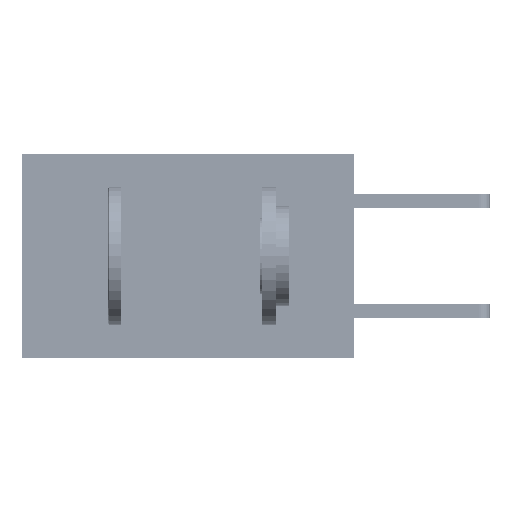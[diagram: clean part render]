
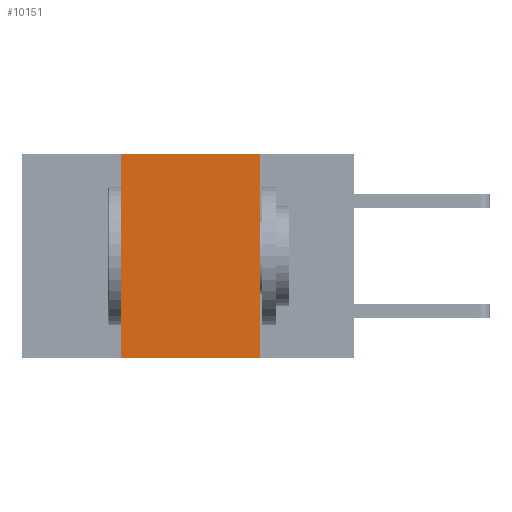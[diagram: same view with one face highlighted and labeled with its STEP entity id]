
A CAD part, left-side view. The second image highlights one B-rep face of the part: STEP entity #10151.
In plain terms, the highlighted planar face has unit normal (-1, 0, 0).
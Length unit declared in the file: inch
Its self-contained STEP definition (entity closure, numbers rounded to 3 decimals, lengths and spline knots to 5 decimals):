
#2378 = LINE ( 'NONE', #46864, #11635 ) ;
#2571 = VECTOR ( 'NONE', #17603, 39.37008 ) ;
#6655 = DIRECTION ( 'NONE',  ( 0., 0., 1. ) ) ;
#6708 = VECTOR ( 'NONE', #42373, 39.37008 ) ;
#7943 = LINE ( 'NONE', #14848, #24016 ) ;
#8687 = AXIS2_PLACEMENT_3D ( 'NONE', #32203, #43185, #32829 ) ;
#9310 = EDGE_CURVE ( 'NONE', #33390, #25339, #2378, .T. ) ;
#10151 = ADVANCED_FACE ( 'NONE', ( #14935 ), #24885, .F. ) ;
#10467 = ORIENTED_EDGE ( 'NONE', *, *, #22022, .F. ) ;
#10662 = CARTESIAN_POINT ( 'NONE',  ( 0., 0.42, 0. ) ) ;
#11635 = VECTOR ( 'NONE', #6655, 39.37008 ) ;
#14848 = CARTESIAN_POINT ( 'NONE',  ( 0., 0.17, 0. ) ) ;
#14935 = FACE_OUTER_BOUND ( 'NONE', #37610, .T. ) ;
#15115 = ORIENTED_EDGE ( 'NONE', *, *, #21054, .F. ) ;
#17018 = CARTESIAN_POINT ( 'NONE',  ( 0., 0.6, 0. ) ) ;
#17603 = DIRECTION ( 'NONE',  ( 0., -1., 0. ) ) ;
#21054 = EDGE_CURVE ( 'NONE', #28473, #40929, #7943, .T. ) ;
#21909 = DIRECTION ( 'NONE',  ( 0., 0., -1. ) ) ;
#22022 = EDGE_CURVE ( 'NONE', #25339, #28473, #27363, .T. ) ;
#24016 = VECTOR ( 'NONE', #21909, 39.37008 ) ;
#24484 = CARTESIAN_POINT ( 'NONE',  ( 0., 0.6, -0.37 ) ) ;
#24885 = PLANE ( 'NONE',  #8687 ) ;
#25339 = VERTEX_POINT ( 'NONE', #10662 ) ;
#27363 = LINE ( 'NONE', #17018, #6708 ) ;
#28473 = VERTEX_POINT ( 'NONE', #30094 ) ;
#29717 = ORIENTED_EDGE ( 'NONE', *, *, #37315, .T. ) ;
#30094 = CARTESIAN_POINT ( 'NONE',  ( 0., 0.17, 0. ) ) ;
#31801 = LINE ( 'NONE', #24484, #2571 ) ;
#32203 = CARTESIAN_POINT ( 'NONE',  ( 0., 0.6, 0. ) ) ;
#32829 = DIRECTION ( 'NONE',  ( 0., 0., -1. ) ) ;
#33390 = VERTEX_POINT ( 'NONE', #35704 ) ;
#34138 = ORIENTED_EDGE ( 'NONE', *, *, #9310, .F. ) ;
#35704 = CARTESIAN_POINT ( 'NONE',  ( 0., 0.42, -0.37 ) ) ;
#37315 = EDGE_CURVE ( 'NONE', #33390, #40929, #31801, .T. ) ;
#37610 = EDGE_LOOP ( 'NONE', ( #15115, #10467, #34138, #29717 ) ) ;
#40929 = VERTEX_POINT ( 'NONE', #45822 ) ;
#42373 = DIRECTION ( 'NONE',  ( 0., -1., 0. ) ) ;
#43185 = DIRECTION ( 'NONE',  ( 1., 0., 0. ) ) ;
#45822 = CARTESIAN_POINT ( 'NONE',  ( 0., 0.17, -0.37 ) ) ;
#46864 = CARTESIAN_POINT ( 'NONE',  ( 0., 0.42, 0. ) ) ;
